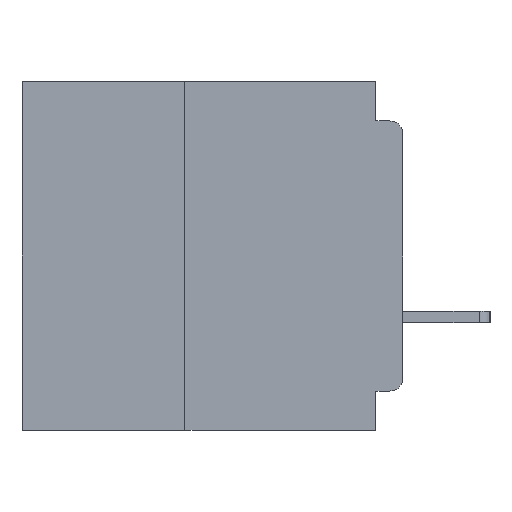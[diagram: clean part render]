
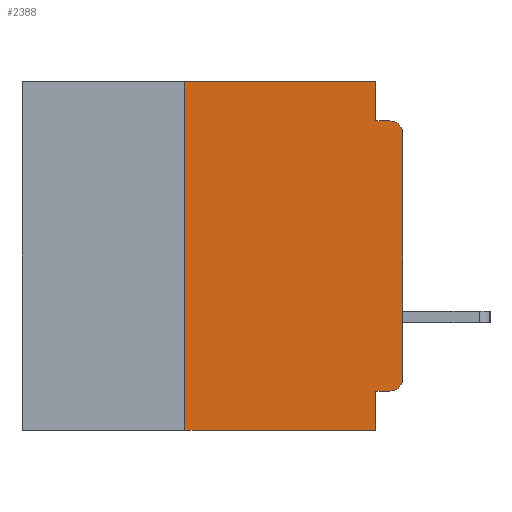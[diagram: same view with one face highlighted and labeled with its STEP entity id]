
A CAD part, left-side view. The second image highlights one B-rep face of the part: STEP entity #2388.
In plain terms, the highlighted planar face has unit normal (-1, 0, 0).
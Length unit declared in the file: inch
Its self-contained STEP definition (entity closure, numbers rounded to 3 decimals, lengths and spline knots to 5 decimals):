
#631 = ORIENTED_EDGE ( 'NONE', *, *, #11046, .F. ) ;
#1188 = VERTEX_POINT ( 'NONE', #23061 ) ;
#1615 = CARTESIAN_POINT ( 'NONE',  ( 0., 0.015, -0.045 ) ) ;
#1908 = AXIS2_PLACEMENT_3D ( 'NONE', #4032, #29688, #7813 ) ;
#2388 = ADVANCED_FACE ( 'NONE', ( #14756 ), #16591, .F. ) ;
#3922 = VECTOR ( 'NONE', #44066, 39.37008 ) ;
#4032 = CARTESIAN_POINT ( 'NONE',  ( 0., 0.015, -0.06 ) ) ;
#4081 = EDGE_CURVE ( 'NONE', #45381, #14038, #18017, .T. ) ;
#4677 = ORIENTED_EDGE ( 'NONE', *, *, #16372, .T. ) ;
#5129 = DIRECTION ( 'NONE',  ( 0., 0., 1. ) ) ;
#5542 = VERTEX_POINT ( 'NONE', #38843 ) ;
#6325 = CARTESIAN_POINT ( 'NONE',  ( 0., 0.015, -0.34 ) ) ;
#6534 = EDGE_CURVE ( 'NONE', #32035, #24981, #27996, .T. ) ;
#7428 = EDGE_CURVE ( 'NONE', #14038, #13617, #46070, .T. ) ;
#7629 = VECTOR ( 'NONE', #5129, 39.37008 ) ;
#7771 = CARTESIAN_POINT ( 'NONE',  ( 0., 0., -0.34 ) ) ;
#7813 = DIRECTION ( 'NONE',  ( 0., 0., -1. ) ) ;
#7858 = CARTESIAN_POINT ( 'NONE',  ( 0., 0.031, -0.045 ) ) ;
#8239 = VECTOR ( 'NONE', #30613, 39.37008 ) ;
#9386 = DIRECTION ( 'NONE',  ( 1., 0., 0. ) ) ;
#10046 = DIRECTION ( 'NONE',  ( 0., 0., -1. ) ) ;
#11046 = EDGE_CURVE ( 'NONE', #1188, #45381, #12345, .T. ) ;
#11186 = ORIENTED_EDGE ( 'NONE', *, *, #26288, .T. ) ;
#12345 = LINE ( 'NONE', #26355, #40332 ) ;
#12890 = ORIENTED_EDGE ( 'NONE', *, *, #4081, .F. ) ;
#13400 = DIRECTION ( 'NONE',  ( 0., -1., 0. ) ) ;
#13617 = VERTEX_POINT ( 'NONE', #1615 ) ;
#13787 = LINE ( 'NONE', #29455, #3922 ) ;
#14038 = VERTEX_POINT ( 'NONE', #7858 ) ;
#14756 = FACE_OUTER_BOUND ( 'NONE', #26719, .T. ) ;
#15968 = CARTESIAN_POINT ( 'NONE',  ( 0., 0.031, 0. ) ) ;
#16084 = CIRCLE ( 'NONE', #1908, 0.015 ) ;
#16372 = EDGE_CURVE ( 'NONE', #25111, #26212, #13787, .T. ) ;
#16591 = PLANE ( 'NONE',  #42494 ) ;
#18017 = LINE ( 'NONE', #15968, #8239 ) ;
#18583 = VECTOR ( 'NONE', #33770, 39.37008 ) ;
#21015 = EDGE_CURVE ( 'NONE', #5542, #21403, #31032, .T. ) ;
#21374 = VECTOR ( 'NONE', #13400, 39.37008 ) ;
#21403 = VERTEX_POINT ( 'NONE', #40916 ) ;
#22473 = ORIENTED_EDGE ( 'NONE', *, *, #29726, .F. ) ;
#23061 = CARTESIAN_POINT ( 'NONE',  ( 0., 0.25, 0. ) ) ;
#23350 = CIRCLE ( 'NONE', #25451, 0.015 ) ;
#24981 = VERTEX_POINT ( 'NONE', #29024 ) ;
#25111 = VERTEX_POINT ( 'NONE', #7771 ) ;
#25451 = AXIS2_PLACEMENT_3D ( 'NONE', #6325, #31897, #10046 ) ;
#25937 = LINE ( 'NONE', #27090, #7629 ) ;
#26212 = VERTEX_POINT ( 'NONE', #43520 ) ;
#26288 = EDGE_CURVE ( 'NONE', #26212, #13617, #16084, .T. ) ;
#26355 = CARTESIAN_POINT ( 'NONE',  ( 0., 0.437, 0. ) ) ;
#26583 = CARTESIAN_POINT ( 'NONE',  ( 0., 0.031, -0.4 ) ) ;
#26719 = EDGE_LOOP ( 'NONE', ( #4677, #11186, #46456, #12890, #631, #22473, #36201, #38457, #37090, #44422 ) ) ;
#27090 = CARTESIAN_POINT ( 'NONE',  ( 0., 0.25, -0.4 ) ) ;
#27572 = EDGE_CURVE ( 'NONE', #32035, #25111, #23350, .T. ) ;
#27916 = VECTOR ( 'NONE', #46257, 39.37008 ) ;
#27996 = LINE ( 'NONE', #30640, #37710 ) ;
#29024 = CARTESIAN_POINT ( 'NONE',  ( 0., 0.031, -0.355 ) ) ;
#29455 = CARTESIAN_POINT ( 'NONE',  ( 0., 0., 0. ) ) ;
#29688 = DIRECTION ( 'NONE',  ( -1., 0., 0. ) ) ;
#29726 = EDGE_CURVE ( 'NONE', #5542, #1188, #25937, .T. ) ;
#30613 = DIRECTION ( 'NONE',  ( 0., 0., -1. ) ) ;
#30640 = CARTESIAN_POINT ( 'NONE',  ( 0., 0., -0.355 ) ) ;
#31032 = LINE ( 'NONE', #38900, #21374 ) ;
#31221 = CARTESIAN_POINT ( 'NONE',  ( 0., 0.437, 0. ) ) ;
#31897 = DIRECTION ( 'NONE',  ( -1., 0., 0. ) ) ;
#32035 = VERTEX_POINT ( 'NONE', #40500 ) ;
#33770 = DIRECTION ( 'NONE',  ( 0., 0., -1. ) ) ;
#34312 = DIRECTION ( 'NONE',  ( 0., 1., 0. ) ) ;
#34922 = DIRECTION ( 'NONE',  ( 0., 0., -1. ) ) ;
#35384 = CARTESIAN_POINT ( 'NONE',  ( 0., 0., -0.045 ) ) ;
#36201 = ORIENTED_EDGE ( 'NONE', *, *, #21015, .T. ) ;
#37090 = ORIENTED_EDGE ( 'NONE', *, *, #6534, .F. ) ;
#37710 = VECTOR ( 'NONE', #34312, 39.37008 ) ;
#38457 = ORIENTED_EDGE ( 'NONE', *, *, #39781, .F. ) ;
#38843 = CARTESIAN_POINT ( 'NONE',  ( 0., 0.25, -0.4 ) ) ;
#38900 = CARTESIAN_POINT ( 'NONE',  ( 0., 0.437, -0.4 ) ) ;
#39781 = EDGE_CURVE ( 'NONE', #24981, #21403, #46399, .T. ) ;
#40332 = VECTOR ( 'NONE', #40675, 39.37008 ) ;
#40500 = CARTESIAN_POINT ( 'NONE',  ( 0., 0.015, -0.355 ) ) ;
#40675 = DIRECTION ( 'NONE',  ( 0., -1., 0. ) ) ;
#40916 = CARTESIAN_POINT ( 'NONE',  ( 0., 0.031, -0.4 ) ) ;
#42494 = AXIS2_PLACEMENT_3D ( 'NONE', #31221, #9386, #34922 ) ;
#43520 = CARTESIAN_POINT ( 'NONE',  ( 0., 0., -0.06 ) ) ;
#44066 = DIRECTION ( 'NONE',  ( 0., 0., 1. ) ) ;
#44422 = ORIENTED_EDGE ( 'NONE', *, *, #27572, .T. ) ;
#44776 = CARTESIAN_POINT ( 'NONE',  ( 0., 0.031, 0. ) ) ;
#45381 = VERTEX_POINT ( 'NONE', #44776 ) ;
#46070 = LINE ( 'NONE', #35384, #27916 ) ;
#46257 = DIRECTION ( 'NONE',  ( 0., -1., 0. ) ) ;
#46399 = LINE ( 'NONE', #26583, #18583 ) ;
#46456 = ORIENTED_EDGE ( 'NONE', *, *, #7428, .F. ) ;
